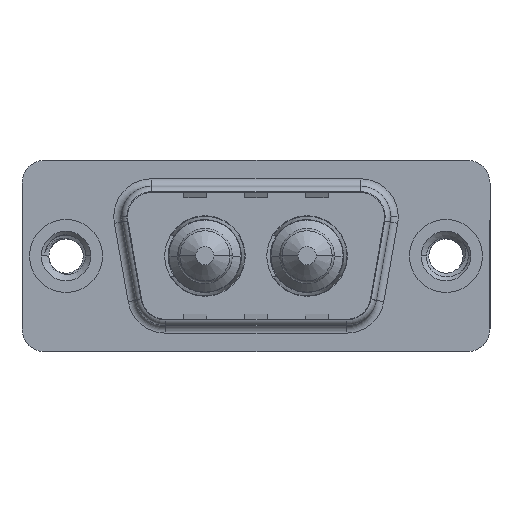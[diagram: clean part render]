
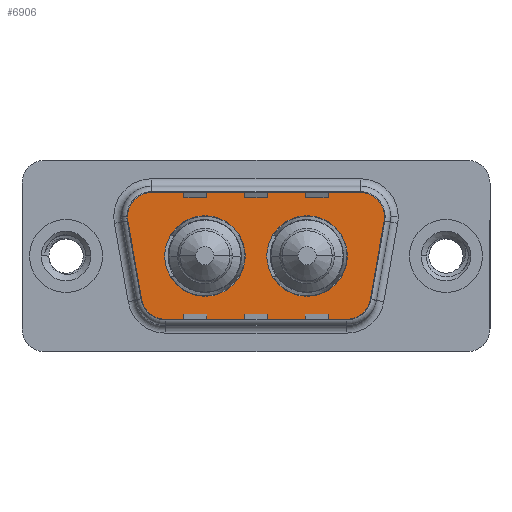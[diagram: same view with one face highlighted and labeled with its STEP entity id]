
A CAD part, top view. The second image highlights one B-rep face of the part: STEP entity #6906.
In plain terms, the highlighted planar face has unit normal (0, 0, 1).
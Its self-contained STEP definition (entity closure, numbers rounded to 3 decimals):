
#90 = EDGE_CURVE ( 'NONE', #9310, #11839, #11887, .T. ) ;
#639 = CARTESIAN_POINT ( 'NONE',  ( 18.541, -2.9, 0. ) ) ;
#654 = AXIS2_PLACEMENT_3D ( 'NONE', #639, #8349, #1757 ) ;
#858 = CARTESIAN_POINT ( 'NONE',  ( 5.436, 2.9, 0. ) ) ;
#1186 = ORIENTED_EDGE ( 'NONE', *, *, #7176, .T. ) ;
#1394 = CARTESIAN_POINT ( 'NONE',  ( 9.14, 0., 0. ) ) ;
#1528 = LINE ( 'NONE', #3605, #7037 ) ;
#1547 = VERTEX_POINT ( 'NONE', #9583 ) ;
#1584 = DIRECTION ( 'NONE',  ( 1., 0., 0. ) ) ;
#1610 = CIRCLE ( 'NONE', #654, 2. ) ;
#1749 = EDGE_CURVE ( 'NONE', #10154, #13368, #4223, .T. ) ;
#1757 = DIRECTION ( 'NONE',  ( 1., 0., 0. ) ) ;
#1837 = EDGE_CURVE ( 'NONE', #8664, #3720, #9414, .T. ) ;
#1852 = CARTESIAN_POINT ( 'NONE',  ( 19.564, 4.9, 0. ) ) ;
#1967 = DIRECTION ( 'NONE',  ( 1., 0., 0. ) ) ;
#2227 = ORIENTED_EDGE ( 'NONE', *, *, #90, .F. ) ;
#2247 = EDGE_CURVE ( 'NONE', #7064, #7808, #5955, .T. ) ;
#2418 = DIRECTION ( 'NONE',  ( 0., 0., 1. ) ) ;
#2504 = DIRECTION ( 'NONE',  ( 1., 0., 0. ) ) ;
#2699 = AXIS2_PLACEMENT_3D ( 'NONE', #2797, #10496, #3881 ) ;
#2705 = VERTEX_POINT ( 'NONE', #3427 ) ;
#2733 = DIRECTION ( 'NONE',  ( 0., 0., 1. ) ) ;
#2789 = ORIENTED_EDGE ( 'NONE', *, *, #1749, .F. ) ;
#2797 = CARTESIAN_POINT ( 'NONE',  ( 19.564, 2.9, 0. ) ) ;
#3033 = VECTOR ( 'NONE', #14213, 1000. ) ;
#3124 = AXIS2_PLACEMENT_3D ( 'NONE', #5663, #2418, #10120 ) ;
#3247 = CARTESIAN_POINT ( 'NONE',  ( 6.459, -2.9, 0. ) ) ;
#3427 = CARTESIAN_POINT ( 'NONE',  ( 4.489, -3.247, 0. ) ) ;
#3450 = DIRECTION ( 'NONE',  ( 0.174, 0.985, 0. ) ) ;
#3605 = CARTESIAN_POINT ( 'NONE',  ( 5.436, 4.9, 0. ) ) ;
#3720 = VERTEX_POINT ( 'NONE', #1852 ) ;
#3841 = CARTESIAN_POINT ( 'NONE',  ( 3.466, 2.553, 0. ) ) ;
#3881 = DIRECTION ( 'NONE',  ( -1., 0., 0. ) ) ;
#4085 = ORIENTED_EDGE ( 'NONE', *, *, #9570, .F. ) ;
#4137 = CIRCLE ( 'NONE', #2699, 2. ) ;
#4223 = CIRCLE ( 'NONE', #6348, 2.65 ) ;
#4267 = VERTEX_POINT ( 'NONE', #3841 ) ;
#4338 = DIRECTION ( 'NONE',  ( -1., 0., 0. ) ) ;
#4461 = ORIENTED_EDGE ( 'NONE', *, *, #1837, .T. ) ;
#4515 = DIRECTION ( 'NONE',  ( 1., 0., 0. ) ) ;
#4535 = DIRECTION ( 'NONE',  ( 0., 0., 1. ) ) ;
#4687 = DIRECTION ( 'NONE',  ( -1., 0., 0. ) ) ;
#5469 = DIRECTION ( 'NONE',  ( 0., 0., 1. ) ) ;
#5497 = ORIENTED_EDGE ( 'NONE', *, *, #13851, .T. ) ;
#5663 = CARTESIAN_POINT ( 'NONE',  ( 18.541, -2.9, 0. ) ) ;
#5955 = LINE ( 'NONE', #12863, #3033 ) ;
#5979 = CARTESIAN_POINT ( 'NONE',  ( 6.459, -4.9, 0. ) ) ;
#6150 = CARTESIAN_POINT ( 'NONE',  ( 19.564, 2.9, 0. ) ) ;
#6185 = VERTEX_POINT ( 'NONE', #12309 ) ;
#6348 = AXIS2_PLACEMENT_3D ( 'NONE', #11088, #2733, #4515 ) ;
#6360 = ORIENTED_EDGE ( 'NONE', *, *, #2247, .T. ) ;
#6465 = EDGE_LOOP ( 'NONE', ( #11180, #2789 ) ) ;
#6518 = CARTESIAN_POINT ( 'NONE',  ( 11.79, 0., 0. ) ) ;
#6526 = ORIENTED_EDGE ( 'NONE', *, *, #7443, .T. ) ;
#6585 = FACE_BOUND ( 'NONE', #14133, .T. ) ;
#6906 = ADVANCED_FACE ( 'NONE', ( #12095, #6585, #12441 ), #9004, .T. ) ;
#7037 = VECTOR ( 'NONE', #4687, 1000. ) ;
#7064 = VERTEX_POINT ( 'NONE', #5979 ) ;
#7176 = EDGE_CURVE ( 'NONE', #7808, #1547, #1610, .T. ) ;
#7443 = EDGE_CURVE ( 'NONE', #4267, #2705, #13808, .T. ) ;
#7778 = CARTESIAN_POINT ( 'NONE',  ( 13.21, 0., 0. ) ) ;
#7808 = VERTEX_POINT ( 'NONE', #9575 ) ;
#8105 = AXIS2_PLACEMENT_3D ( 'NONE', #12048, #5469, #13154 ) ;
#8338 = CARTESIAN_POINT ( 'NONE',  ( 21.564, 2.9, 0. ) ) ;
#8349 = DIRECTION ( 'NONE',  ( 0., 0., 1. ) ) ;
#8394 = CARTESIAN_POINT ( 'NONE',  ( 21.534, 2.553, 0. ) ) ;
#8559 = DIRECTION ( 'NONE',  ( 0., 0., 1. ) ) ;
#8567 = DIRECTION ( 'NONE',  ( -1., 0., 0. ) ) ;
#8664 = VERTEX_POINT ( 'NONE', #8338 ) ;
#8813 = LINE ( 'NONE', #11166, #12068 ) ;
#8897 = EDGE_CURVE ( 'NONE', #13368, #10154, #14158, .T. ) ;
#8997 = ORIENTED_EDGE ( 'NONE', *, *, #11549, .T. ) ;
#9004 = PLANE ( 'NONE',  #3124 ) ;
#9089 = DIRECTION ( 'NONE',  ( 0., 0., 1. ) ) ;
#9145 = ORIENTED_EDGE ( 'NONE', *, *, #13333, .T. ) ;
#9180 = EDGE_CURVE ( 'NONE', #6185, #4267, #13657, .T. ) ;
#9310 = VERTEX_POINT ( 'NONE', #6518 ) ;
#9414 = CIRCLE ( 'NONE', #13746, 2. ) ;
#9570 = EDGE_CURVE ( 'NONE', #11839, #9310, #13814, .T. ) ;
#9575 = CARTESIAN_POINT ( 'NONE',  ( 18.541, -4.9, 0. ) ) ;
#9583 = CARTESIAN_POINT ( 'NONE',  ( 20.511, -3.247, 0. ) ) ;
#9743 = CARTESIAN_POINT ( 'NONE',  ( 6.49, 0., 0. ) ) ;
#10120 = DIRECTION ( 'NONE',  ( 1., 0., 0. ) ) ;
#10154 = VERTEX_POINT ( 'NONE', #7778 ) ;
#10181 = ORIENTED_EDGE ( 'NONE', *, *, #9180, .T. ) ;
#10259 = CARTESIAN_POINT ( 'NONE',  ( 18.51, 0., 0. ) ) ;
#10496 = DIRECTION ( 'NONE',  ( 0., 0., 1. ) ) ;
#10556 = VECTOR ( 'NONE', #11916, 1000. ) ;
#10956 = DIRECTION ( 'NONE',  ( 0., 0., 1. ) ) ;
#11022 = DIRECTION ( 'NONE',  ( 0., 0., 1. ) ) ;
#11088 = CARTESIAN_POINT ( 'NONE',  ( 15.86, 0., 0. ) ) ;
#11166 = CARTESIAN_POINT ( 'NONE',  ( 21.534, 2.553, 0. ) ) ;
#11180 = ORIENTED_EDGE ( 'NONE', *, *, #8897, .F. ) ;
#11269 = AXIS2_PLACEMENT_3D ( 'NONE', #3247, #10956, #4338 ) ;
#11320 = EDGE_CURVE ( 'NONE', #1547, #14149, #8813, .T. ) ;
#11549 = EDGE_CURVE ( 'NONE', #14149, #8664, #4137, .T. ) ;
#11661 = CARTESIAN_POINT ( 'NONE',  ( 9.14, 0., 0. ) ) ;
#11839 = VERTEX_POINT ( 'NONE', #9743 ) ;
#11887 = CIRCLE ( 'NONE', #13157, 2.65 ) ;
#11916 = DIRECTION ( 'NONE',  ( 0.174, -0.985, 0. ) ) ;
#11952 = AXIS2_PLACEMENT_3D ( 'NONE', #1394, #9089, #2504 ) ;
#12048 = CARTESIAN_POINT ( 'NONE',  ( 15.86, 0., 0. ) ) ;
#12068 = VECTOR ( 'NONE', #3450, 1000. ) ;
#12095 = FACE_BOUND ( 'NONE', #6465, .T. ) ;
#12309 = CARTESIAN_POINT ( 'NONE',  ( 5.436, 4.9, 0. ) ) ;
#12441 = FACE_OUTER_BOUND ( 'NONE', #12615, .T. ) ;
#12615 = EDGE_LOOP ( 'NONE', ( #1186, #14221, #8997, #4461, #9145, #10181, #6526, #5497, #6360 ) ) ;
#12863 = CARTESIAN_POINT ( 'NONE',  ( 6.459, -4.9, 0. ) ) ;
#12950 = AXIS2_PLACEMENT_3D ( 'NONE', #858, #8559, #1967 ) ;
#12963 = CARTESIAN_POINT ( 'NONE',  ( 3.466, 2.553, 0. ) ) ;
#13154 = DIRECTION ( 'NONE',  ( 1., 0., 0. ) ) ;
#13157 = AXIS2_PLACEMENT_3D ( 'NONE', #11661, #4535, #1584 ) ;
#13333 = EDGE_CURVE ( 'NONE', #3720, #6185, #1528, .T. ) ;
#13368 = VERTEX_POINT ( 'NONE', #10259 ) ;
#13657 = CIRCLE ( 'NONE', #12950, 2. ) ;
#13746 = AXIS2_PLACEMENT_3D ( 'NONE', #6150, #11022, #8567 ) ;
#13808 = LINE ( 'NONE', #12963, #10556 ) ;
#13814 = CIRCLE ( 'NONE', #11952, 2.65 ) ;
#13851 = EDGE_CURVE ( 'NONE', #2705, #7064, #13878, .T. ) ;
#13878 = CIRCLE ( 'NONE', #11269, 2. ) ;
#14133 = EDGE_LOOP ( 'NONE', ( #2227, #4085 ) ) ;
#14149 = VERTEX_POINT ( 'NONE', #8394 ) ;
#14158 = CIRCLE ( 'NONE', #8105, 2.65 ) ;
#14213 = DIRECTION ( 'NONE',  ( 1., 0., 0. ) ) ;
#14221 = ORIENTED_EDGE ( 'NONE', *, *, #11320, .T. ) ;
